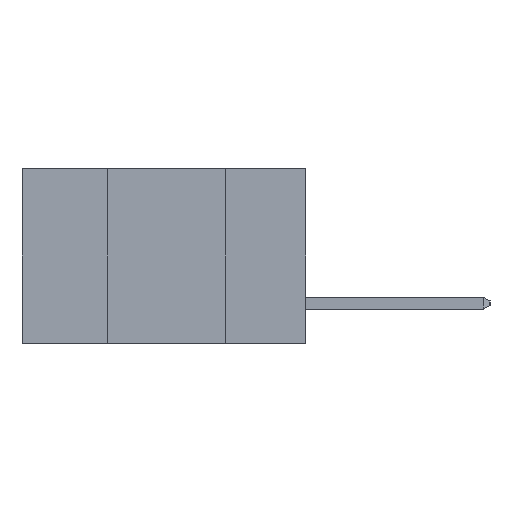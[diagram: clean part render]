
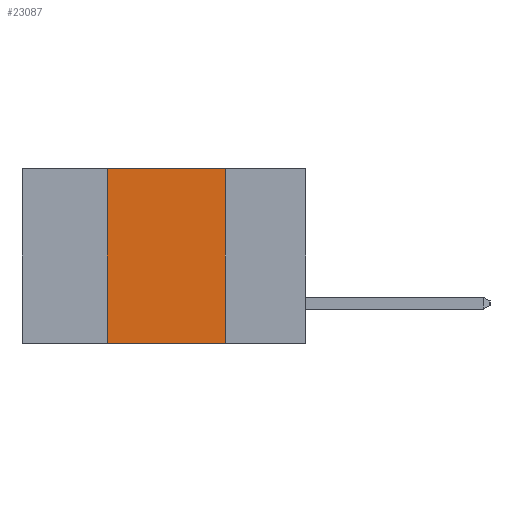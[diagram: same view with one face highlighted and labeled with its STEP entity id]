
A CAD part, left-side view. The second image highlights one B-rep face of the part: STEP entity #23087.
In plain terms, the highlighted planar face has unit normal (-1, 0, 0).
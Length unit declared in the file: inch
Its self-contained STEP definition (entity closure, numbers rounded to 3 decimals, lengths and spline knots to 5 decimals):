
#56 = AXIS2_PLACEMENT_3D ( 'NONE', #25338, #3144, #18725 ) ;
#882 = PLANE ( 'NONE',  #56 ) ;
#1084 = CARTESIAN_POINT ( 'NONE',  ( 0., 0.6, 0. ) ) ;
#1630 = FACE_OUTER_BOUND ( 'NONE', #23878, .T. ) ;
#2002 = CARTESIAN_POINT ( 'NONE',  ( 0., 0.42, 0. ) ) ;
#2182 = CARTESIAN_POINT ( 'NONE',  ( 0., 0.17, -0.37 ) ) ;
#3144 = DIRECTION ( 'NONE',  ( 1., 0., 0. ) ) ;
#4349 = LINE ( 'NONE', #1084, #26624 ) ;
#4780 = VERTEX_POINT ( 'NONE', #18580 ) ;
#5103 = LINE ( 'NONE', #2002, #28079 ) ;
#5566 = VECTOR ( 'NONE', #24546, 39.37008 ) ;
#5611 = VERTEX_POINT ( 'NONE', #6577 ) ;
#6262 = VERTEX_POINT ( 'NONE', #2182 ) ;
#6577 = CARTESIAN_POINT ( 'NONE',  ( 0., 0.42, -0.37 ) ) ;
#6712 = CARTESIAN_POINT ( 'NONE',  ( 0., 0.6, -0.37 ) ) ;
#8498 = ORIENTED_EDGE ( 'NONE', *, *, #11485, .F. ) ;
#9267 = LINE ( 'NONE', #21276, #26326 ) ;
#9927 = ORIENTED_EDGE ( 'NONE', *, *, #10012, .T. ) ;
#10012 = EDGE_CURVE ( 'NONE', #5611, #6262, #24694, .T. ) ;
#11485 = EDGE_CURVE ( 'NONE', #5611, #4780, #5103, .T. ) ;
#13201 = DIRECTION ( 'NONE',  ( 0., 0., 1. ) ) ;
#16346 = VERTEX_POINT ( 'NONE', #28221 ) ;
#18580 = CARTESIAN_POINT ( 'NONE',  ( 0., 0.42, 0. ) ) ;
#18725 = DIRECTION ( 'NONE',  ( 0., 0., -1. ) ) ;
#18906 = DIRECTION ( 'NONE',  ( 0., -1., 0. ) ) ;
#19634 = ORIENTED_EDGE ( 'NONE', *, *, #21023, .F. ) ;
#20441 = EDGE_CURVE ( 'NONE', #16346, #6262, #9267, .T. ) ;
#21023 = EDGE_CURVE ( 'NONE', #4780, #16346, #4349, .T. ) ;
#21276 = CARTESIAN_POINT ( 'NONE',  ( 0., 0.17, 0. ) ) ;
#23087 = ADVANCED_FACE ( 'NONE', ( #1630 ), #882, .F. ) ;
#23454 = ORIENTED_EDGE ( 'NONE', *, *, #20441, .F. ) ;
#23493 = DIRECTION ( 'NONE',  ( 0., 0., -1. ) ) ;
#23878 = EDGE_LOOP ( 'NONE', ( #23454, #19634, #8498, #9927 ) ) ;
#24546 = DIRECTION ( 'NONE',  ( 0., -1., 0. ) ) ;
#24694 = LINE ( 'NONE', #6712, #5566 ) ;
#25338 = CARTESIAN_POINT ( 'NONE',  ( 0., 0.6, 0. ) ) ;
#26326 = VECTOR ( 'NONE', #23493, 39.37008 ) ;
#26624 = VECTOR ( 'NONE', #18906, 39.37008 ) ;
#28079 = VECTOR ( 'NONE', #13201, 39.37008 ) ;
#28221 = CARTESIAN_POINT ( 'NONE',  ( 0., 0.17, 0. ) ) ;
